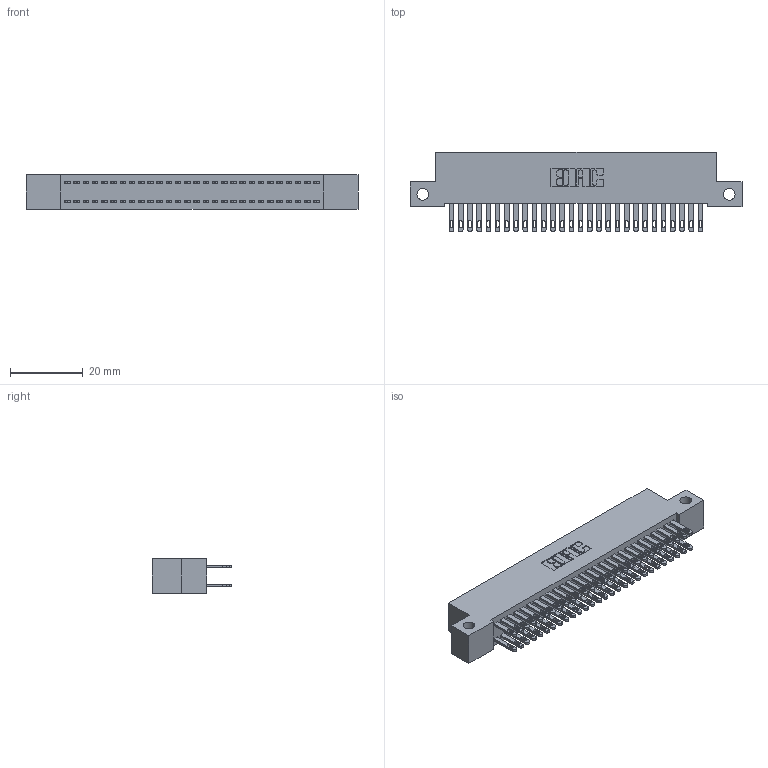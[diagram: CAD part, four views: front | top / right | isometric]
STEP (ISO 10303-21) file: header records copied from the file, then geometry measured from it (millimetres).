
FILE_DESCRIPTION (( 'STEP AP203' ), '1' );
FILE_NAME ('892-056-500-212.STEP', '2020-09-21T18:47:21', ( '' ), ( '' ), 'SwSTEP 2.0', 'SolidWorks 2020', '' );
FILE_SCHEMA (( 'CONFIG_CONTROL_DESIGN' ));
Length unit declared in the file: inch
Products named in the file (3): 892-056-500-212; 842 Part_Side Mount; 345-292-001_345-293-100
Assembly tree (57 placements, depth 2):
  892-056-500-212
    842 Part_Side Mount
    345-292-001_345-293-100  x56
Bounding box: 91.44 x 21.85 x 9.4 mm (x, y, z)
Volume: 8246.8 mm3; surface area: 13455.2 mm2
Topology: 57 solids, 57 shells, 2798 faces, 8531 edges, 5686 vertices
Faces by surface type: plane 1746, cylinder 1052
Entity records: 19625 total; most frequent: CARTESIAN_POINT 3266, ORIENTED_EDGE 3202, DIRECTION 2817, EDGE_CURVE 1601, VECTOR 1469, LINE 1469, VERTEX_POINT 1066, AXIS2_PLACEMENT_3D 674
